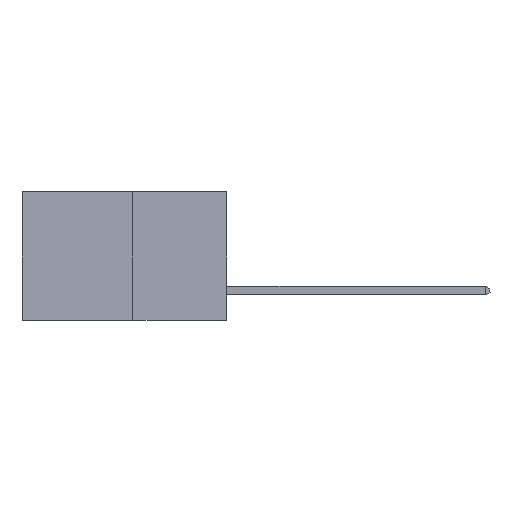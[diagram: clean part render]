
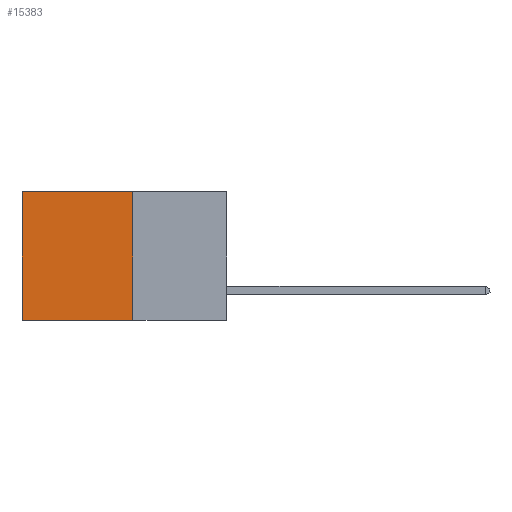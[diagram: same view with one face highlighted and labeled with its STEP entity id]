
A CAD part, left-side view. The second image highlights one B-rep face of the part: STEP entity #15383.
In plain terms, the highlighted planar face has unit normal (-1, 0, 0).
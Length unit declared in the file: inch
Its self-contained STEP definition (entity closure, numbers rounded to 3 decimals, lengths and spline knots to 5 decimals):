
#65 = CARTESIAN_POINT ( 'NONE',  ( 0.277, 0.27, 0. ) ) ;
#383 = CARTESIAN_POINT ( 'NONE',  ( 0.277, 0.27, -0.37 ) ) ;
#2344 = PLANE ( 'NONE',  #4981 ) ;
#2387 = VERTEX_POINT ( 'NONE', #65 ) ;
#2827 = ORIENTED_EDGE ( 'NONE', *, *, #15989, .T. ) ;
#3094 = LINE ( 'NONE', #383, #7257 ) ;
#3275 = VECTOR ( 'NONE', #14709, 39.37008 ) ;
#3584 = CARTESIAN_POINT ( 'NONE',  ( 0.277, 0.59, -0.37 ) ) ;
#3641 = DIRECTION ( 'NONE',  ( 0., 0., -1. ) ) ;
#3721 = LINE ( 'NONE', #17221, #3275 ) ;
#4309 = EDGE_CURVE ( 'NONE', #2387, #15556, #3721, .T. ) ;
#4981 = AXIS2_PLACEMENT_3D ( 'NONE', #7973, #17740, #9354 ) ;
#5546 = CARTESIAN_POINT ( 'NONE',  ( 0.277, 0.59, 0. ) ) ;
#6209 = EDGE_LOOP ( 'NONE', ( #2827, #8597, #17098, #8783 ) ) ;
#7103 = LINE ( 'NONE', #15709, #14516 ) ;
#7257 = VECTOR ( 'NONE', #10201, 39.37008 ) ;
#7386 = DIRECTION ( 'NONE',  ( 0., 0., -1. ) ) ;
#7647 = VECTOR ( 'NONE', #3641, 39.37008 ) ;
#7973 = CARTESIAN_POINT ( 'NONE',  ( 0.277, 0.27, -0.37 ) ) ;
#8597 = ORIENTED_EDGE ( 'NONE', *, *, #11965, .F. ) ;
#8783 = ORIENTED_EDGE ( 'NONE', *, *, #4309, .T. ) ;
#9354 = DIRECTION ( 'NONE',  ( 0., 0., -1. ) ) ;
#10101 = EDGE_CURVE ( 'NONE', #2387, #12282, #7103, .T. ) ;
#10201 = DIRECTION ( 'NONE',  ( 0., 1., 0. ) ) ;
#10982 = VERTEX_POINT ( 'NONE', #16467 ) ;
#11777 = LINE ( 'NONE', #3584, #7647 ) ;
#11965 = EDGE_CURVE ( 'NONE', #12282, #10982, #3094, .T. ) ;
#12259 = CARTESIAN_POINT ( 'NONE',  ( 0.277, 0.27, -0.37 ) ) ;
#12282 = VERTEX_POINT ( 'NONE', #12259 ) ;
#14516 = VECTOR ( 'NONE', #7386, 39.37008 ) ;
#14709 = DIRECTION ( 'NONE',  ( 0., 1., 0. ) ) ;
#15383 = ADVANCED_FACE ( 'NONE', ( #18148 ), #2344, .F. ) ;
#15556 = VERTEX_POINT ( 'NONE', #5546 ) ;
#15709 = CARTESIAN_POINT ( 'NONE',  ( 0.277, 0.27, -0.37 ) ) ;
#15989 = EDGE_CURVE ( 'NONE', #15556, #10982, #11777, .T. ) ;
#16467 = CARTESIAN_POINT ( 'NONE',  ( 0.277, 0.59, -0.37 ) ) ;
#17098 = ORIENTED_EDGE ( 'NONE', *, *, #10101, .F. ) ;
#17221 = CARTESIAN_POINT ( 'NONE',  ( 0.277, 0.27, 0. ) ) ;
#17740 = DIRECTION ( 'NONE',  ( 1., 0., 0. ) ) ;
#18148 = FACE_OUTER_BOUND ( 'NONE', #6209, .T. ) ;
